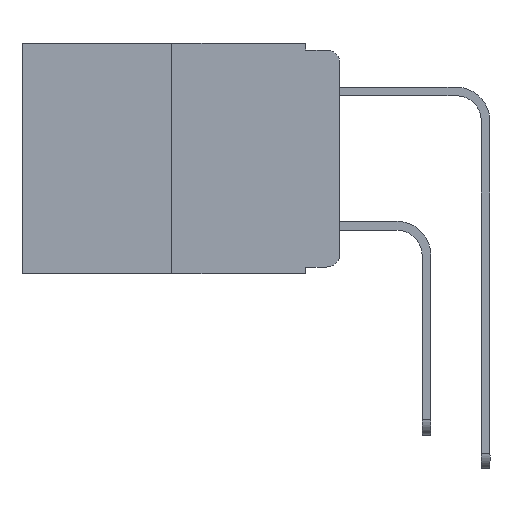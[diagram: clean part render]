
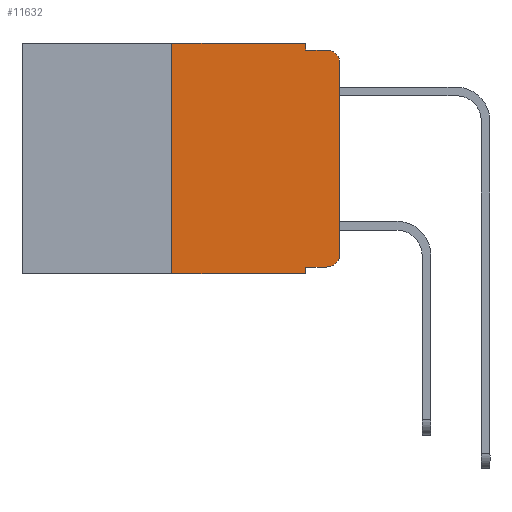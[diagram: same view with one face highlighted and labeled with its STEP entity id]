
A CAD part, left-side view. The second image highlights one B-rep face of the part: STEP entity #11632.
In plain terms, the highlighted planar face has unit normal (-1, 0, 0).
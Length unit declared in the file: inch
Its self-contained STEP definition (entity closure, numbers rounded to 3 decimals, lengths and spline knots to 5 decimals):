
#6 = EDGE_CURVE ( 'NONE', #404, #10288, #5436, .T. ) ;
#166 = LINE ( 'NONE', #4192, #8459 ) ;
#172 = VERTEX_POINT ( 'NONE', #1766 ) ;
#404 = VERTEX_POINT ( 'NONE', #3400 ) ;
#570 = ORIENTED_EDGE ( 'NONE', *, *, #6, .T. ) ;
#904 = DIRECTION ( 'NONE',  ( 1., 0., 0. ) ) ;
#925 = LINE ( 'NONE', #4653, #8339 ) ;
#1310 = ORIENTED_EDGE ( 'NONE', *, *, #1727, .F. ) ;
#1387 = VECTOR ( 'NONE', #10222, 39.37008 ) ;
#1410 = DIRECTION ( 'NONE',  ( 0., 0., -1. ) ) ;
#1482 = ORIENTED_EDGE ( 'NONE', *, *, #10970, .F. ) ;
#1727 = EDGE_CURVE ( 'NONE', #3696, #12240, #12642, .T. ) ;
#1766 = CARTESIAN_POINT ( 'NONE',  ( 0., 0.051, -0.333 ) ) ;
#1776 = VERTEX_POINT ( 'NONE', #1940 ) ;
#1940 = CARTESIAN_POINT ( 'NONE',  ( 0., 0.051, 0. ) ) ;
#2092 = EDGE_CURVE ( 'NONE', #4317, #2432, #8586, .T. ) ;
#2118 = CARTESIAN_POINT ( 'NONE',  ( 0., 0.25, 0. ) ) ;
#2432 = VERTEX_POINT ( 'NONE', #7533 ) ;
#2780 = AXIS2_PLACEMENT_3D ( 'NONE', #5720, #9800, #7972 ) ;
#3091 = ORIENTED_EDGE ( 'NONE', *, *, #4744, .F. ) ;
#3243 = EDGE_CURVE ( 'NONE', #8088, #404, #12328, .T. ) ;
#3400 = CARTESIAN_POINT ( 'NONE',  ( 0., 0., -0.313 ) ) ;
#3642 = FACE_OUTER_BOUND ( 'NONE', #11108, .T. ) ;
#3696 = VERTEX_POINT ( 'NONE', #5324 ) ;
#3798 = DIRECTION ( 'NONE',  ( 0., 0., -1. ) ) ;
#3998 = VECTOR ( 'NONE', #10597, 39.37008 ) ;
#4178 = DIRECTION ( 'NONE',  ( 0., 0., -1. ) ) ;
#4192 = CARTESIAN_POINT ( 'NONE',  ( 0., 0.473, 0. ) ) ;
#4317 = VERTEX_POINT ( 'NONE', #10756 ) ;
#4465 = CARTESIAN_POINT ( 'NONE',  ( 0., 0.25, 0. ) ) ;
#4643 = VECTOR ( 'NONE', #12386, 39.37008 ) ;
#4653 = CARTESIAN_POINT ( 'NONE',  ( 0., 0.051, 0. ) ) ;
#4744 = EDGE_CURVE ( 'NONE', #1776, #3696, #925, .T. ) ;
#5012 = DIRECTION ( 'NONE',  ( -1., 0., 0. ) ) ;
#5159 = CARTESIAN_POINT ( 'NONE',  ( 0., 0.02, -0.333 ) ) ;
#5186 = EDGE_CURVE ( 'NONE', #4317, #8527, #7381, .T. ) ;
#5214 = CARTESIAN_POINT ( 'NONE',  ( 0., 0.02, -0.313 ) ) ;
#5324 = CARTESIAN_POINT ( 'NONE',  ( 0., 0.051, -0.01 ) ) ;
#5360 = CARTESIAN_POINT ( 'NONE',  ( 0., 0.051, -0.333 ) ) ;
#5436 = LINE ( 'NONE', #11199, #1387 ) ;
#5720 = CARTESIAN_POINT ( 'NONE',  ( 0., 0.02, -0.03 ) ) ;
#5744 = CARTESIAN_POINT ( 'NONE',  ( 0., 0.051, -0.01 ) ) ;
#5840 = ORIENTED_EDGE ( 'NONE', *, *, #5186, .F. ) ;
#6089 = AXIS2_PLACEMENT_3D ( 'NONE', #5214, #5012, #4178 ) ;
#6124 = VECTOR ( 'NONE', #9630, 39.37008 ) ;
#6576 = CARTESIAN_POINT ( 'NONE',  ( 0., 0.02, -0.01 ) ) ;
#6714 = CIRCLE ( 'NONE', #2780, 0.02 ) ;
#6763 = EDGE_CURVE ( 'NONE', #8527, #1776, #166, .T. ) ;
#6837 = ORIENTED_EDGE ( 'NONE', *, *, #7500, .T. ) ;
#6900 = ORIENTED_EDGE ( 'NONE', *, *, #2092, .T. ) ;
#6927 = EDGE_CURVE ( 'NONE', #172, #8088, #11312, .T. ) ;
#7381 = LINE ( 'NONE', #4465, #4643 ) ;
#7500 = EDGE_CURVE ( 'NONE', #10288, #12240, #6714, .T. ) ;
#7533 = CARTESIAN_POINT ( 'NONE',  ( 0., 0.051, -0.343 ) ) ;
#7554 = LINE ( 'NONE', #9426, #9077 ) ;
#7683 = CARTESIAN_POINT ( 'NONE',  ( 0., 0.473, -0.343 ) ) ;
#7972 = DIRECTION ( 'NONE',  ( 0., 0., -1. ) ) ;
#8088 = VERTEX_POINT ( 'NONE', #5159 ) ;
#8339 = VECTOR ( 'NONE', #3798, 39.37008 ) ;
#8459 = VECTOR ( 'NONE', #9115, 39.37008 ) ;
#8495 = AXIS2_PLACEMENT_3D ( 'NONE', #9743, #904, #11759 ) ;
#8527 = VERTEX_POINT ( 'NONE', #2118 ) ;
#8586 = LINE ( 'NONE', #7683, #3998 ) ;
#8776 = PLANE ( 'NONE',  #8495 ) ;
#8984 = VECTOR ( 'NONE', #9240, 39.37008 ) ;
#9077 = VECTOR ( 'NONE', #1410, 39.37008 ) ;
#9115 = DIRECTION ( 'NONE',  ( 0., -1., 0. ) ) ;
#9240 = DIRECTION ( 'NONE',  ( 0., -1., 0. ) ) ;
#9426 = CARTESIAN_POINT ( 'NONE',  ( 0., 0.051, 0. ) ) ;
#9630 = DIRECTION ( 'NONE',  ( 0., -1., 0. ) ) ;
#9743 = CARTESIAN_POINT ( 'NONE',  ( 0., 0.473, 0. ) ) ;
#9800 = DIRECTION ( 'NONE',  ( -1., 0., 0. ) ) ;
#10213 = ORIENTED_EDGE ( 'NONE', *, *, #3243, .T. ) ;
#10222 = DIRECTION ( 'NONE',  ( 0., 0., 1. ) ) ;
#10288 = VERTEX_POINT ( 'NONE', #10633 ) ;
#10597 = DIRECTION ( 'NONE',  ( 0., -1., 0. ) ) ;
#10633 = CARTESIAN_POINT ( 'NONE',  ( 0., 0., -0.03 ) ) ;
#10756 = CARTESIAN_POINT ( 'NONE',  ( 0., 0.25, -0.343 ) ) ;
#10970 = EDGE_CURVE ( 'NONE', #172, #2432, #7554, .T. ) ;
#11108 = EDGE_LOOP ( 'NONE', ( #570, #6837, #1310, #3091, #12203, #5840, #6900, #1482, #12380, #10213 ) ) ;
#11199 = CARTESIAN_POINT ( 'NONE',  ( 0., 0., 0. ) ) ;
#11312 = LINE ( 'NONE', #5360, #8984 ) ;
#11632 = ADVANCED_FACE ( 'NONE', ( #3642 ), #8776, .F. ) ;
#11759 = DIRECTION ( 'NONE',  ( 0., 0., -1. ) ) ;
#12203 = ORIENTED_EDGE ( 'NONE', *, *, #6763, .F. ) ;
#12240 = VERTEX_POINT ( 'NONE', #6576 ) ;
#12328 = CIRCLE ( 'NONE', #6089, 0.02 ) ;
#12380 = ORIENTED_EDGE ( 'NONE', *, *, #6927, .T. ) ;
#12386 = DIRECTION ( 'NONE',  ( 0., 0., 1. ) ) ;
#12642 = LINE ( 'NONE', #5744, #6124 ) ;
